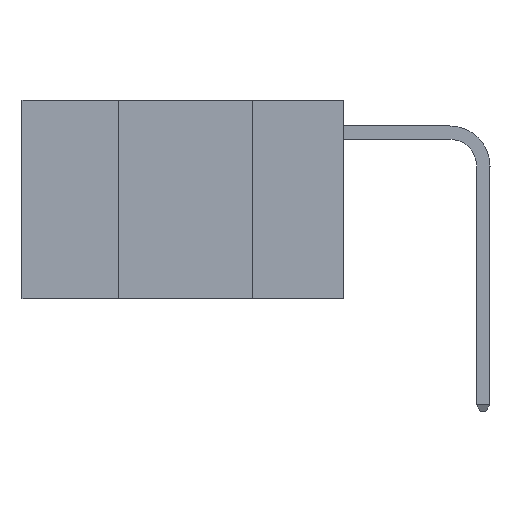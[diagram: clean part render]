
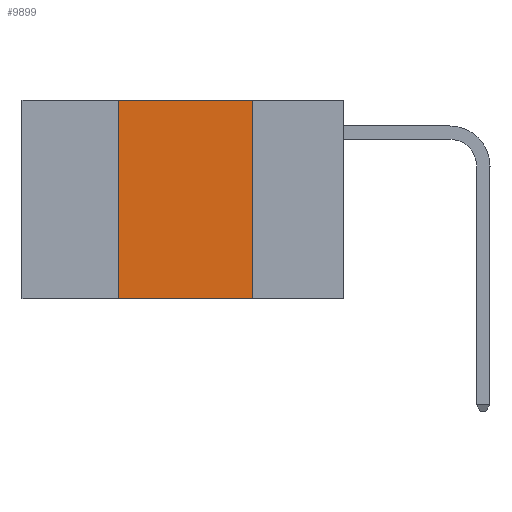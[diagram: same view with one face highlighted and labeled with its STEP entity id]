
A CAD part, left-side view. The second image highlights one B-rep face of the part: STEP entity #9899.
In plain terms, the highlighted planar face has unit normal (-1, 0, 0).
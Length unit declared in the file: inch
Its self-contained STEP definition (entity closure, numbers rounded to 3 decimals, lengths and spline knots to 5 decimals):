
#538 = PLANE ( 'NONE',  #7114 ) ;
#899 = VERTEX_POINT ( 'NONE', #11431 ) ;
#1254 = ORIENTED_EDGE ( 'NONE', *, *, #9838, .F. ) ;
#1530 = LINE ( 'NONE', #2001, #9512 ) ;
#2001 = CARTESIAN_POINT ( 'NONE',  ( 0., 0.6, 0. ) ) ;
#2446 = VERTEX_POINT ( 'NONE', #4119 ) ;
#3259 = CARTESIAN_POINT ( 'NONE',  ( 0., 0.42, -0.37 ) ) ;
#3595 = LINE ( 'NONE', #11459, #6046 ) ;
#3808 = DIRECTION ( 'NONE',  ( 1., 0., 0. ) ) ;
#3867 = LINE ( 'NONE', #12177, #11608 ) ;
#4119 = CARTESIAN_POINT ( 'NONE',  ( 0., 0.42, 0. ) ) ;
#4439 = ORIENTED_EDGE ( 'NONE', *, *, #12525, .F. ) ;
#4676 = CARTESIAN_POINT ( 'NONE',  ( 0., 0.17, 0. ) ) ;
#5084 = ORIENTED_EDGE ( 'NONE', *, *, #8593, .F. ) ;
#5421 = DIRECTION ( 'NONE',  ( 0., 0., 1. ) ) ;
#6046 = VECTOR ( 'NONE', #5421, 39.37008 ) ;
#7114 = AXIS2_PLACEMENT_3D ( 'NONE', #11822, #3808, #10944 ) ;
#7274 = VERTEX_POINT ( 'NONE', #9733 ) ;
#7989 = VERTEX_POINT ( 'NONE', #3259 ) ;
#8593 = EDGE_CURVE ( 'NONE', #7989, #2446, #3595, .T. ) ;
#8852 = DIRECTION ( 'NONE',  ( 0., 0., -1. ) ) ;
#9451 = EDGE_LOOP ( 'NONE', ( #1254, #4439, #5084, #10210 ) ) ;
#9512 = VECTOR ( 'NONE', #10280, 39.37008 ) ;
#9733 = CARTESIAN_POINT ( 'NONE',  ( 0., 0.17, -0.37 ) ) ;
#9835 = VECTOR ( 'NONE', #8852, 39.37008 ) ;
#9838 = EDGE_CURVE ( 'NONE', #899, #7274, #12313, .T. ) ;
#9899 = ADVANCED_FACE ( 'NONE', ( #11199 ), #538, .F. ) ;
#10210 = ORIENTED_EDGE ( 'NONE', *, *, #11104, .T. ) ;
#10280 = DIRECTION ( 'NONE',  ( 0., -1., 0. ) ) ;
#10944 = DIRECTION ( 'NONE',  ( 0., 0., -1. ) ) ;
#11104 = EDGE_CURVE ( 'NONE', #7989, #7274, #3867, .T. ) ;
#11199 = FACE_OUTER_BOUND ( 'NONE', #9451, .T. ) ;
#11431 = CARTESIAN_POINT ( 'NONE',  ( 0., 0.17, 0. ) ) ;
#11459 = CARTESIAN_POINT ( 'NONE',  ( 0., 0.42, 0. ) ) ;
#11608 = VECTOR ( 'NONE', #13064, 39.37008 ) ;
#11822 = CARTESIAN_POINT ( 'NONE',  ( 0., 0.6, 0. ) ) ;
#12177 = CARTESIAN_POINT ( 'NONE',  ( 0., 0.6, -0.37 ) ) ;
#12313 = LINE ( 'NONE', #4676, #9835 ) ;
#12525 = EDGE_CURVE ( 'NONE', #2446, #899, #1530, .T. ) ;
#13064 = DIRECTION ( 'NONE',  ( 0., -1., 0. ) ) ;
